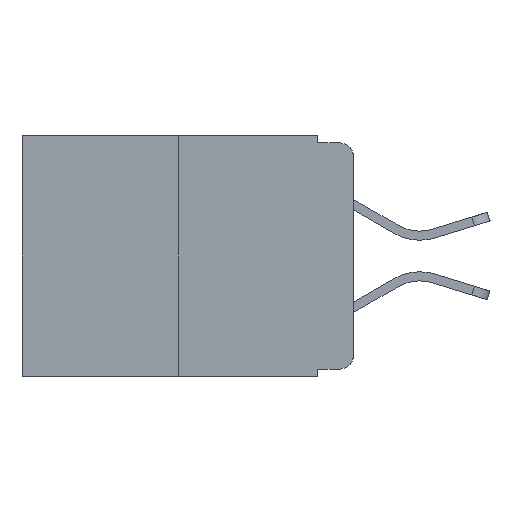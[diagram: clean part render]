
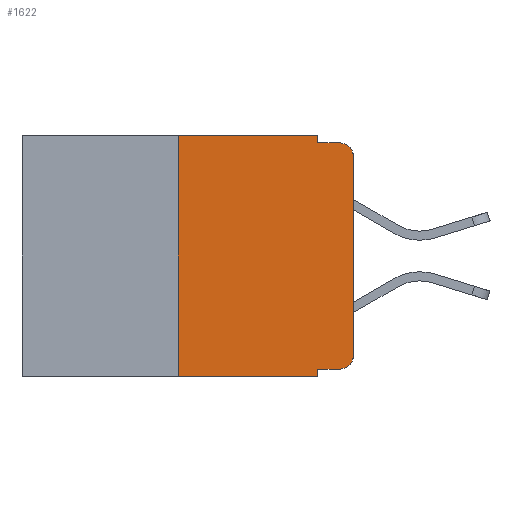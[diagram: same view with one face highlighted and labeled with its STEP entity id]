
A CAD part, left-side view. The second image highlights one B-rep face of the part: STEP entity #1622.
In plain terms, the highlighted planar face has unit normal (-1, 0, 0).
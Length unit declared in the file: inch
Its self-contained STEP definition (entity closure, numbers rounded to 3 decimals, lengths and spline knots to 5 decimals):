
#77 = EDGE_CURVE ( 'NONE', #1689, #14323, #3741, .T. ) ;
#294 = VERTEX_POINT ( 'NONE', #11236 ) ;
#345 = LINE ( 'NONE', #12860, #3351 ) ;
#497 = CARTESIAN_POINT ( 'NONE',  ( 0., 0.051, -0.01 ) ) ;
#552 = DIRECTION ( 'NONE',  ( 0., 0., -1. ) ) ;
#700 = EDGE_LOOP ( 'NONE', ( #6934, #5984, #2769, #6680, #14550, #9730, #14136, #12550, #9429, #5601 ) ) ;
#755 = DIRECTION ( 'NONE',  ( 0., 0., 1. ) ) ;
#940 = EDGE_CURVE ( 'NONE', #14190, #14323, #4107, .T. ) ;
#1163 = CARTESIAN_POINT ( 'NONE',  ( 0., 0., 0. ) ) ;
#1469 = VECTOR ( 'NONE', #4855, 39.37008 ) ;
#1586 = CARTESIAN_POINT ( 'NONE',  ( 0., 0.25, 0. ) ) ;
#1622 = ADVANCED_FACE ( 'NONE', ( #3888 ), #6468, .F. ) ;
#1689 = VERTEX_POINT ( 'NONE', #3644 ) ;
#1767 = VERTEX_POINT ( 'NONE', #11448 ) ;
#1780 = EDGE_CURVE ( 'NONE', #2719, #14190, #4891, .T. ) ;
#1844 = CARTESIAN_POINT ( 'NONE',  ( 0., 0.051, 0. ) ) ;
#1898 = CARTESIAN_POINT ( 'NONE',  ( 0., 0.25, -0.343 ) ) ;
#2032 = CARTESIAN_POINT ( 'NONE',  ( 0., 0.051, -0.01 ) ) ;
#2066 = DIRECTION ( 'NONE',  ( 0., -1., 0. ) ) ;
#2112 = CARTESIAN_POINT ( 'NONE',  ( 0., 0.02, -0.01 ) ) ;
#2719 = VERTEX_POINT ( 'NONE', #1844 ) ;
#2769 = ORIENTED_EDGE ( 'NONE', *, *, #940, .F. ) ;
#2843 = VECTOR ( 'NONE', #2066, 39.37008 ) ;
#2878 = DIRECTION ( 'NONE',  ( 0., 0., 1. ) ) ;
#3039 = LINE ( 'NONE', #9842, #15328 ) ;
#3123 = AXIS2_PLACEMENT_3D ( 'NONE', #6343, #5434, #5468 ) ;
#3351 = VECTOR ( 'NONE', #7036, 39.37008 ) ;
#3510 = EDGE_CURVE ( 'NONE', #7268, #1689, #7474, .T. ) ;
#3644 = CARTESIAN_POINT ( 'NONE',  ( 0., 0., -0.03 ) ) ;
#3741 = CIRCLE ( 'NONE', #15066, 0.02 ) ;
#3836 = EDGE_CURVE ( 'NONE', #294, #7268, #14677, .T. ) ;
#3888 = FACE_OUTER_BOUND ( 'NONE', #700, .T. ) ;
#4107 = LINE ( 'NONE', #2032, #7081 ) ;
#4135 = CARTESIAN_POINT ( 'NONE',  ( 0., 0., -0.313 ) ) ;
#4855 = DIRECTION ( 'NONE',  ( 0., 0., -1. ) ) ;
#4891 = LINE ( 'NONE', #12614, #1469 ) ;
#5050 = VECTOR ( 'NONE', #5598, 39.37008 ) ;
#5434 = DIRECTION ( 'NONE',  ( -1., 0., 0. ) ) ;
#5449 = LINE ( 'NONE', #5538, #5050 ) ;
#5468 = DIRECTION ( 'NONE',  ( 0., 0., -1. ) ) ;
#5538 = CARTESIAN_POINT ( 'NONE',  ( 0., 0.473, -0.343 ) ) ;
#5598 = DIRECTION ( 'NONE',  ( 0., -1., 0. ) ) ;
#5601 = ORIENTED_EDGE ( 'NONE', *, *, #3836, .T. ) ;
#5611 = LINE ( 'NONE', #1586, #11523 ) ;
#5984 = ORIENTED_EDGE ( 'NONE', *, *, #77, .T. ) ;
#6321 = EDGE_CURVE ( 'NONE', #8822, #11877, #5449, .T. ) ;
#6343 = CARTESIAN_POINT ( 'NONE',  ( 0., 0.02, -0.313 ) ) ;
#6468 = PLANE ( 'NONE',  #10013 ) ;
#6680 = ORIENTED_EDGE ( 'NONE', *, *, #1780, .F. ) ;
#6934 = ORIENTED_EDGE ( 'NONE', *, *, #3510, .T. ) ;
#7036 = DIRECTION ( 'NONE',  ( 0., 0., -1. ) ) ;
#7081 = VECTOR ( 'NONE', #9020, 39.37008 ) ;
#7268 = VERTEX_POINT ( 'NONE', #4135 ) ;
#7474 = LINE ( 'NONE', #1163, #13274 ) ;
#8026 = EDGE_CURVE ( 'NONE', #8822, #1767, #5611, .T. ) ;
#8822 = VERTEX_POINT ( 'NONE', #1898 ) ;
#8839 = EDGE_CURVE ( 'NONE', #14935, #11877, #345, .T. ) ;
#9020 = DIRECTION ( 'NONE',  ( 0., -1., 0. ) ) ;
#9337 = DIRECTION ( 'NONE',  ( 1., 0., 0. ) ) ;
#9429 = ORIENTED_EDGE ( 'NONE', *, *, #15105, .T. ) ;
#9441 = LINE ( 'NONE', #14095, #2843 ) ;
#9730 = ORIENTED_EDGE ( 'NONE', *, *, #8026, .F. ) ;
#9801 = CARTESIAN_POINT ( 'NONE',  ( 0., 0.02, -0.03 ) ) ;
#9842 = CARTESIAN_POINT ( 'NONE',  ( 0., 0.051, -0.333 ) ) ;
#10013 = AXIS2_PLACEMENT_3D ( 'NONE', #10374, #9337, #552 ) ;
#10374 = CARTESIAN_POINT ( 'NONE',  ( 0., 0.473, 0. ) ) ;
#11236 = CARTESIAN_POINT ( 'NONE',  ( 0., 0.02, -0.333 ) ) ;
#11448 = CARTESIAN_POINT ( 'NONE',  ( 0., 0.25, 0. ) ) ;
#11523 = VECTOR ( 'NONE', #2878, 39.37008 ) ;
#11860 = CARTESIAN_POINT ( 'NONE',  ( 0., 0.051, -0.333 ) ) ;
#11877 = VERTEX_POINT ( 'NONE', #14033 ) ;
#12169 = DIRECTION ( 'NONE',  ( 0., -1., 0. ) ) ;
#12291 = DIRECTION ( 'NONE',  ( 0., 0., -1. ) ) ;
#12550 = ORIENTED_EDGE ( 'NONE', *, *, #8839, .F. ) ;
#12614 = CARTESIAN_POINT ( 'NONE',  ( 0., 0.051, 0. ) ) ;
#12860 = CARTESIAN_POINT ( 'NONE',  ( 0., 0.051, 0. ) ) ;
#13220 = DIRECTION ( 'NONE',  ( -1., 0., 0. ) ) ;
#13274 = VECTOR ( 'NONE', #755, 39.37008 ) ;
#14033 = CARTESIAN_POINT ( 'NONE',  ( 0., 0.051, -0.343 ) ) ;
#14095 = CARTESIAN_POINT ( 'NONE',  ( 0., 0.473, 0. ) ) ;
#14136 = ORIENTED_EDGE ( 'NONE', *, *, #6321, .T. ) ;
#14190 = VERTEX_POINT ( 'NONE', #497 ) ;
#14323 = VERTEX_POINT ( 'NONE', #2112 ) ;
#14550 = ORIENTED_EDGE ( 'NONE', *, *, #15338, .F. ) ;
#14677 = CIRCLE ( 'NONE', #3123, 0.02 ) ;
#14935 = VERTEX_POINT ( 'NONE', #11860 ) ;
#15066 = AXIS2_PLACEMENT_3D ( 'NONE', #9801, #13220, #12291 ) ;
#15105 = EDGE_CURVE ( 'NONE', #14935, #294, #3039, .T. ) ;
#15328 = VECTOR ( 'NONE', #12169, 39.37008 ) ;
#15338 = EDGE_CURVE ( 'NONE', #1767, #2719, #9441, .T. ) ;
